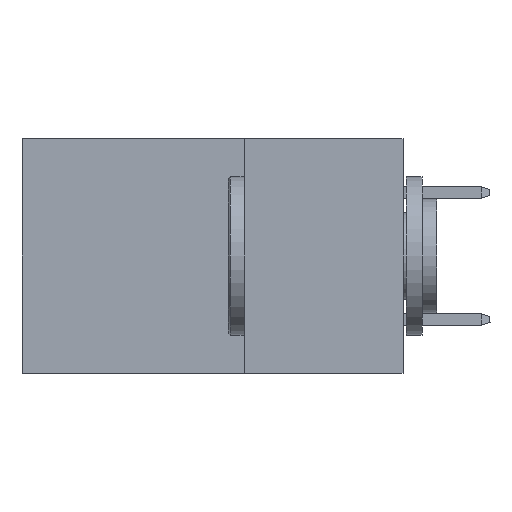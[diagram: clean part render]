
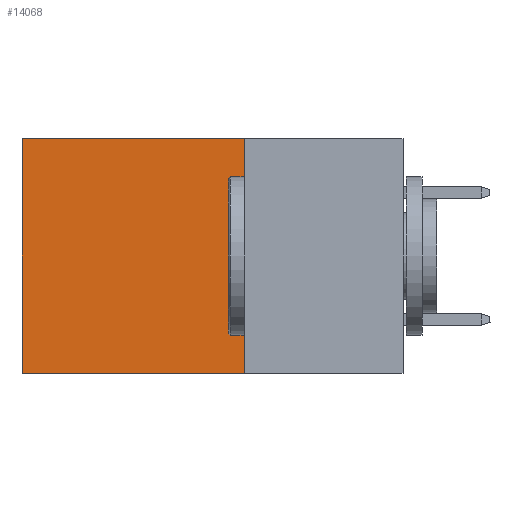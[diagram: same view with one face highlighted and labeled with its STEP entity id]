
A CAD part, left-side view. The second image highlights one B-rep face of the part: STEP entity #14068.
In plain terms, the highlighted planar face has unit normal (-1, 0, 0).
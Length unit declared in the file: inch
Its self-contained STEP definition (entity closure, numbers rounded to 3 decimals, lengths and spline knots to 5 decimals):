
#207 = AXIS2_PLACEMENT_3D ( 'NONE', #21828, #1230, #17769 ) ;
#505 = EDGE_CURVE ( 'NONE', #24774, #12271, #17337, .T. ) ;
#591 = CARTESIAN_POINT ( 'NONE',  ( 0.2875, 0.25, 0. ) ) ;
#988 = VERTEX_POINT ( 'NONE', #22498 ) ;
#1181 = DIRECTION ( 'NONE',  ( 0., 1., 0. ) ) ;
#1190 = LINE ( 'NONE', #15200, #6377 ) ;
#1230 = DIRECTION ( 'NONE',  ( 1., 0., 0. ) ) ;
#1675 = ORIENTED_EDGE ( 'NONE', *, *, #18432, .F. ) ;
#3124 = EDGE_CURVE ( 'NONE', #5012, #988, #1190, .T. ) ;
#3328 = VECTOR ( 'NONE', #25950, 39.37008 ) ;
#4570 = ORIENTED_EDGE ( 'NONE', *, *, #20127, .T. ) ;
#4944 = CARTESIAN_POINT ( 'NONE',  ( 0.2875, 0.25, 0. ) ) ;
#5012 = VERTEX_POINT ( 'NONE', #24607 ) ;
#5396 = PLANE ( 'NONE',  #207 ) ;
#6377 = VECTOR ( 'NONE', #7522, 39.37008 ) ;
#7522 = DIRECTION ( 'NONE',  ( 0., 1., 0. ) ) ;
#7534 = DIRECTION ( 'NONE',  ( 0., 0., -1. ) ) ;
#9471 = CARTESIAN_POINT ( 'NONE',  ( 0.2875, 0.6, 0. ) ) ;
#9748 = ORIENTED_EDGE ( 'NONE', *, *, #505, .T. ) ;
#10104 = CARTESIAN_POINT ( 'NONE',  ( 0.2875, 0.25, 0. ) ) ;
#12271 = VERTEX_POINT ( 'NONE', #9471 ) ;
#13338 = FACE_OUTER_BOUND ( 'NONE', #14506, .T. ) ;
#14068 = ADVANCED_FACE ( 'NONE', ( #13338 ), #5396, .F. ) ;
#14202 = ORIENTED_EDGE ( 'NONE', *, *, #3124, .F. ) ;
#14506 = EDGE_LOOP ( 'NONE', ( #4570, #14202, #1675, #9748 ) ) ;
#15200 = CARTESIAN_POINT ( 'NONE',  ( 0.2875, 0.25, -0.37 ) ) ;
#15732 = CARTESIAN_POINT ( 'NONE',  ( 0.2875, 0.6, 0. ) ) ;
#16266 = LINE ( 'NONE', #15732, #18032 ) ;
#17337 = LINE ( 'NONE', #4944, #17975 ) ;
#17769 = DIRECTION ( 'NONE',  ( 0., 0., -1. ) ) ;
#17975 = VECTOR ( 'NONE', #1181, 39.37008 ) ;
#18032 = VECTOR ( 'NONE', #7534, 39.37008 ) ;
#18432 = EDGE_CURVE ( 'NONE', #24774, #5012, #22090, .T. ) ;
#20127 = EDGE_CURVE ( 'NONE', #12271, #988, #16266, .T. ) ;
#21828 = CARTESIAN_POINT ( 'NONE',  ( 0.2875, 0.25, 0. ) ) ;
#22090 = LINE ( 'NONE', #10104, #3328 ) ;
#22498 = CARTESIAN_POINT ( 'NONE',  ( 0.2875, 0.6, -0.37 ) ) ;
#24607 = CARTESIAN_POINT ( 'NONE',  ( 0.2875, 0.25, -0.37 ) ) ;
#24774 = VERTEX_POINT ( 'NONE', #591 ) ;
#25950 = DIRECTION ( 'NONE',  ( 0., 0., -1. ) ) ;
